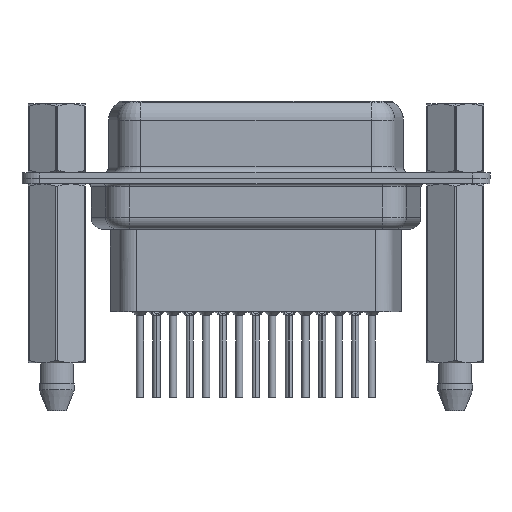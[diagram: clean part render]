
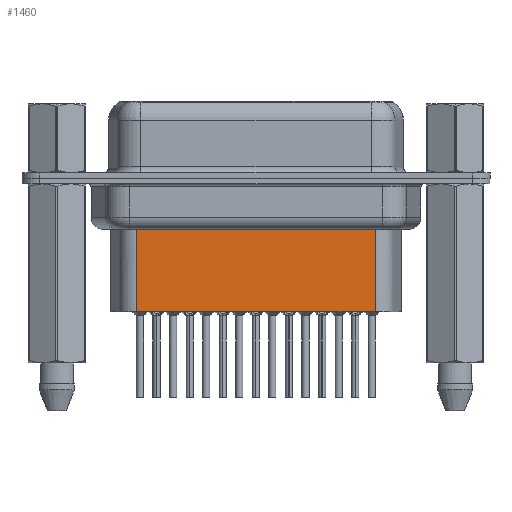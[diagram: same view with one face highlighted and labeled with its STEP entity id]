
A CAD part, front view. The second image highlights one B-rep face of the part: STEP entity #1460.
In plain terms, the highlighted planar face has unit normal (0, -1, 0).
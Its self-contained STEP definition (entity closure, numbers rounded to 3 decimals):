
#294 = CARTESIAN_POINT ( 'NONE',  ( 6.681, -3.5, -4.097 ) ) ;
#1171 = VERTEX_POINT ( 'NONE', #12901 ) ;
#1213 = ORIENTED_EDGE ( 'NONE', *, *, #8171, .T. ) ;
#1276 = DIRECTION ( 'NONE',  ( 0., 0., -1. ) ) ;
#1460 = ADVANCED_FACE ( 'NONE', ( #25630 ), #6698, .T. ) ;
#4928 = ORIENTED_EDGE ( 'NONE', *, *, #12008, .F. ) ;
#5485 = LINE ( 'NONE', #22275, #25020 ) ;
#6223 = LINE ( 'NONE', #18306, #19817 ) ;
#6698 = PLANE ( 'NONE',  #9237 ) ;
#8171 = EDGE_CURVE ( 'NONE', #26958, #22729, #17755, .T. ) ;
#9237 = AXIS2_PLACEMENT_3D ( 'NONE', #28050, #18186, #12426 ) ;
#10809 = CARTESIAN_POINT ( 'NONE',  ( 6.681, -3.5, -3.1 ) ) ;
#12008 = EDGE_CURVE ( 'NONE', #23628, #22729, #5485, .T. ) ;
#12246 = CARTESIAN_POINT ( 'NONE',  ( 26.619, -3.5, -11.15 ) ) ;
#12426 = DIRECTION ( 'NONE',  ( 1., 0., 0. ) ) ;
#12901 = CARTESIAN_POINT ( 'NONE',  ( 26.619, -3.5, -4.097 ) ) ;
#14204 = ORIENTED_EDGE ( 'NONE', *, *, #15703, .T. ) ;
#14987 = VECTOR ( 'NONE', #1276, 1000. ) ;
#15703 = EDGE_CURVE ( 'NONE', #1171, #26958, #18713, .T. ) ;
#16526 = EDGE_CURVE ( 'NONE', #1171, #23628, #6223, .T. ) ;
#16962 = VECTOR ( 'NONE', #22808, 1000. ) ;
#17755 = LINE ( 'NONE', #10809, #14987 ) ;
#17852 = DIRECTION ( 'NONE',  ( 0., 0., -1. ) ) ;
#18186 = DIRECTION ( 'NONE',  ( 0., -1., 0. ) ) ;
#18306 = CARTESIAN_POINT ( 'NONE',  ( 26.619, -3.5, -3.1 ) ) ;
#18713 = LINE ( 'NONE', #27983, #16962 ) ;
#19199 = ORIENTED_EDGE ( 'NONE', *, *, #16526, .F. ) ;
#19418 = DIRECTION ( 'NONE',  ( -1., 0., 0. ) ) ;
#19817 = VECTOR ( 'NONE', #17852, 1000. ) ;
#21523 = CARTESIAN_POINT ( 'NONE',  ( 6.681, -3.5, -11.15 ) ) ;
#21906 = EDGE_LOOP ( 'NONE', ( #19199, #14204, #1213, #4928 ) ) ;
#22275 = CARTESIAN_POINT ( 'NONE',  ( 6.681, -3.5, -11.15 ) ) ;
#22729 = VERTEX_POINT ( 'NONE', #21523 ) ;
#22808 = DIRECTION ( 'NONE',  ( -1., 0., 0. ) ) ;
#23628 = VERTEX_POINT ( 'NONE', #12246 ) ;
#25020 = VECTOR ( 'NONE', #19418, 1000. ) ;
#25630 = FACE_OUTER_BOUND ( 'NONE', #21906, .T. ) ;
#26958 = VERTEX_POINT ( 'NONE', #294 ) ;
#27983 = CARTESIAN_POINT ( 'NONE',  ( 6.434, -3.5, -4.097 ) ) ;
#28050 = CARTESIAN_POINT ( 'NONE',  ( 6.681, -3.5, -3.1 ) ) ;
